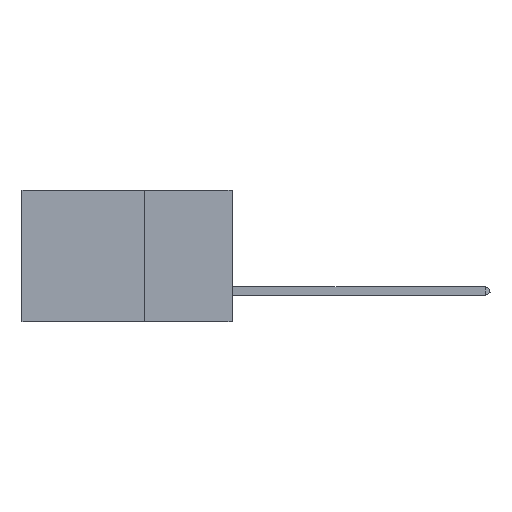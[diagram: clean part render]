
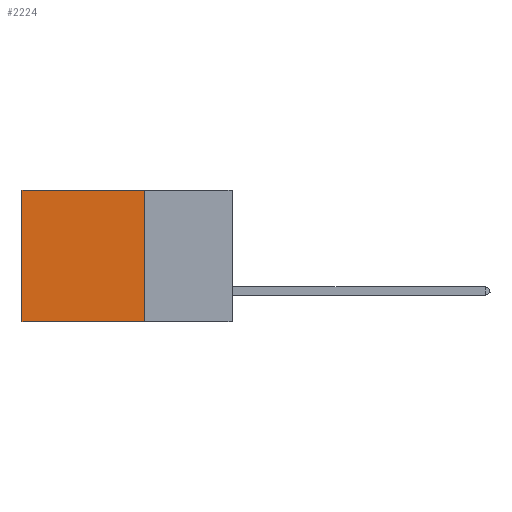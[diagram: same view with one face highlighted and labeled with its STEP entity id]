
A CAD part, left-side view. The second image highlights one B-rep face of the part: STEP entity #2224.
In plain terms, the highlighted planar face has unit normal (-1, 0, 0).
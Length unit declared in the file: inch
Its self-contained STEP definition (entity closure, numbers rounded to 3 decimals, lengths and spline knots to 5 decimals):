
#983 = CARTESIAN_POINT ( 'NONE',  ( 0.2875, 0.6, -0.375 ) ) ;
#1477 = DIRECTION ( 'NONE',  ( 0., 0., -1. ) ) ;
#1958 = CARTESIAN_POINT ( 'NONE',  ( 0.2875, 0.6, 0. ) ) ;
#2224 = ADVANCED_FACE ( 'NONE', ( #5899 ), #5998, .F. ) ;
#2873 = LINE ( 'NONE', #13786, #14374 ) ;
#2951 = CARTESIAN_POINT ( 'NONE',  ( 0.2875, 0.25, 0. ) ) ;
#3341 = DIRECTION ( 'NONE',  ( 0., 1., 0. ) ) ;
#3776 = CARTESIAN_POINT ( 'NONE',  ( 0.2875, 0.25, -0.375 ) ) ;
#3816 = LINE ( 'NONE', #6169, #6514 ) ;
#4822 = AXIS2_PLACEMENT_3D ( 'NONE', #8357, #10690, #1477 ) ;
#5390 = ORIENTED_EDGE ( 'NONE', *, *, #9416, .T. ) ;
#5537 = EDGE_CURVE ( 'NONE', #8776, #8705, #11811, .T. ) ;
#5561 = CARTESIAN_POINT ( 'NONE',  ( 0.2875, 0.25, -0.375 ) ) ;
#5692 = VECTOR ( 'NONE', #9588, 39.37008 ) ;
#5899 = FACE_OUTER_BOUND ( 'NONE', #6726, .T. ) ;
#5998 = PLANE ( 'NONE',  #4822 ) ;
#6030 = CARTESIAN_POINT ( 'NONE',  ( 0.2875, 0.25, -0.375 ) ) ;
#6169 = CARTESIAN_POINT ( 'NONE',  ( 0.2875, 0.25, 0. ) ) ;
#6514 = VECTOR ( 'NONE', #8576, 39.37008 ) ;
#6535 = VERTEX_POINT ( 'NONE', #1958 ) ;
#6726 = EDGE_LOOP ( 'NONE', ( #5390, #10656, #12901, #12266 ) ) ;
#7030 = VECTOR ( 'NONE', #3341, 39.37008 ) ;
#7815 = EDGE_CURVE ( 'NONE', #8776, #6535, #3816, .T. ) ;
#8357 = CARTESIAN_POINT ( 'NONE',  ( 0.2875, 0.25, -0.375 ) ) ;
#8576 = DIRECTION ( 'NONE',  ( 0., 1., 0. ) ) ;
#8705 = VERTEX_POINT ( 'NONE', #3776 ) ;
#8776 = VERTEX_POINT ( 'NONE', #2951 ) ;
#9416 = EDGE_CURVE ( 'NONE', #6535, #10148, #2873, .T. ) ;
#9588 = DIRECTION ( 'NONE',  ( 0., 0., -1. ) ) ;
#10080 = LINE ( 'NONE', #5561, #7030 ) ;
#10148 = VERTEX_POINT ( 'NONE', #983 ) ;
#10189 = DIRECTION ( 'NONE',  ( 0., 0., -1. ) ) ;
#10656 = ORIENTED_EDGE ( 'NONE', *, *, #14660, .F. ) ;
#10690 = DIRECTION ( 'NONE',  ( 1., 0., 0. ) ) ;
#11811 = LINE ( 'NONE', #6030, #5692 ) ;
#12266 = ORIENTED_EDGE ( 'NONE', *, *, #7815, .T. ) ;
#12901 = ORIENTED_EDGE ( 'NONE', *, *, #5537, .F. ) ;
#13786 = CARTESIAN_POINT ( 'NONE',  ( 0.2875, 0.6, -0.375 ) ) ;
#14374 = VECTOR ( 'NONE', #10189, 39.37008 ) ;
#14660 = EDGE_CURVE ( 'NONE', #8705, #10148, #10080, .T. ) ;
